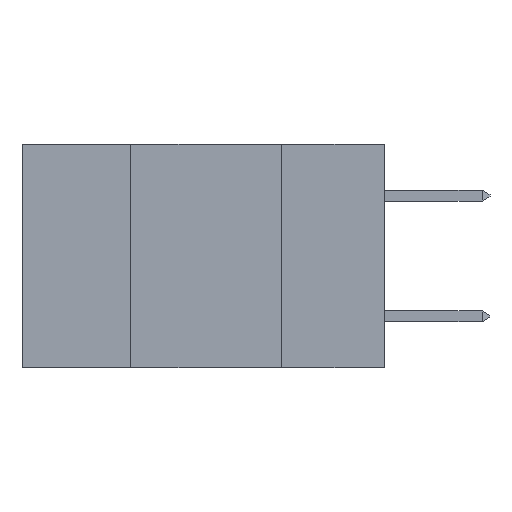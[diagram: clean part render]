
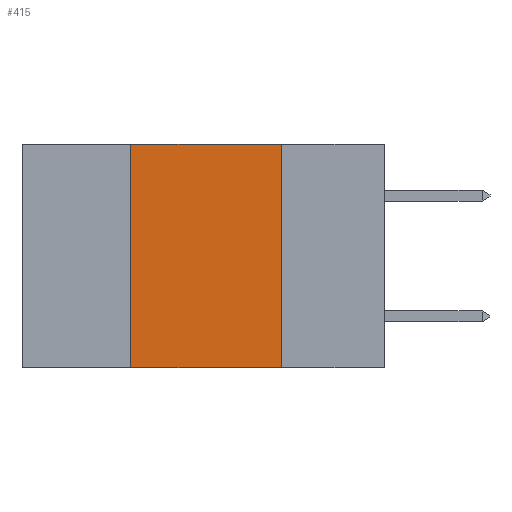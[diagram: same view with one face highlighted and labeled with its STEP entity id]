
A CAD part, left-side view. The second image highlights one B-rep face of the part: STEP entity #415.
In plain terms, the highlighted planar face has unit normal (-1, 0, 0).
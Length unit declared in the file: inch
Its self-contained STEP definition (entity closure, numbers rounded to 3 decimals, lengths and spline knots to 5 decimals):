
#58 = EDGE_CURVE ( 'NONE', #7162, #1908, #7741, .T. ) ;
#286 = PLANE ( 'NONE',  #1630 ) ;
#415 = ADVANCED_FACE ( 'NONE', ( #7683 ), #286, .F. ) ;
#643 = ORIENTED_EDGE ( 'NONE', *, *, #3153, .F. ) ;
#1168 = ORIENTED_EDGE ( 'NONE', *, *, #3556, .T. ) ;
#1630 = AXIS2_PLACEMENT_3D ( 'NONE', #1742, #9261, #1927 ) ;
#1742 = CARTESIAN_POINT ( 'NONE',  ( 0., 0.6, 0. ) ) ;
#1749 = EDGE_LOOP ( 'NONE', ( #2159, #643, #2950, #1168 ) ) ;
#1908 = VERTEX_POINT ( 'NONE', #4761 ) ;
#1927 = DIRECTION ( 'NONE',  ( 0., 0., -1. ) ) ;
#2000 = CARTESIAN_POINT ( 'NONE',  ( 0., 0.42, -0.37 ) ) ;
#2048 = DIRECTION ( 'NONE',  ( 0., 0., -1. ) ) ;
#2159 = ORIENTED_EDGE ( 'NONE', *, *, #7127, .F. ) ;
#2950 = ORIENTED_EDGE ( 'NONE', *, *, #58, .F. ) ;
#3153 = EDGE_CURVE ( 'NONE', #1908, #3343, #4900, .T. ) ;
#3343 = VERTEX_POINT ( 'NONE', #6794 ) ;
#3446 = VECTOR ( 'NONE', #5827, 39.37008 ) ;
#3556 = EDGE_CURVE ( 'NONE', #7162, #9524, #8392, .T. ) ;
#3692 = CARTESIAN_POINT ( 'NONE',  ( 0., 0.42, 0. ) ) ;
#4166 = CARTESIAN_POINT ( 'NONE',  ( 0., 0.6, -0.37 ) ) ;
#4334 = LINE ( 'NONE', #9427, #8609 ) ;
#4410 = CARTESIAN_POINT ( 'NONE',  ( 0., 0.17, -0.37 ) ) ;
#4761 = CARTESIAN_POINT ( 'NONE',  ( 0., 0.42, 0. ) ) ;
#4900 = LINE ( 'NONE', #7097, #8171 ) ;
#5575 = DIRECTION ( 'NONE',  ( 0., -1., 0. ) ) ;
#5827 = DIRECTION ( 'NONE',  ( 0., 0., 1. ) ) ;
#5849 = VECTOR ( 'NONE', #5575, 39.37008 ) ;
#6794 = CARTESIAN_POINT ( 'NONE',  ( 0., 0.17, 0. ) ) ;
#7097 = CARTESIAN_POINT ( 'NONE',  ( 0., 0.6, 0. ) ) ;
#7127 = EDGE_CURVE ( 'NONE', #3343, #9524, #4334, .T. ) ;
#7162 = VERTEX_POINT ( 'NONE', #2000 ) ;
#7683 = FACE_OUTER_BOUND ( 'NONE', #1749, .T. ) ;
#7741 = LINE ( 'NONE', #3692, #3446 ) ;
#8171 = VECTOR ( 'NONE', #8592, 39.37008 ) ;
#8392 = LINE ( 'NONE', #4166, #5849 ) ;
#8592 = DIRECTION ( 'NONE',  ( 0., -1., 0. ) ) ;
#8609 = VECTOR ( 'NONE', #2048, 39.37008 ) ;
#9261 = DIRECTION ( 'NONE',  ( 1., 0., 0. ) ) ;
#9427 = CARTESIAN_POINT ( 'NONE',  ( 0., 0.17, 0. ) ) ;
#9524 = VERTEX_POINT ( 'NONE', #4410 ) ;
